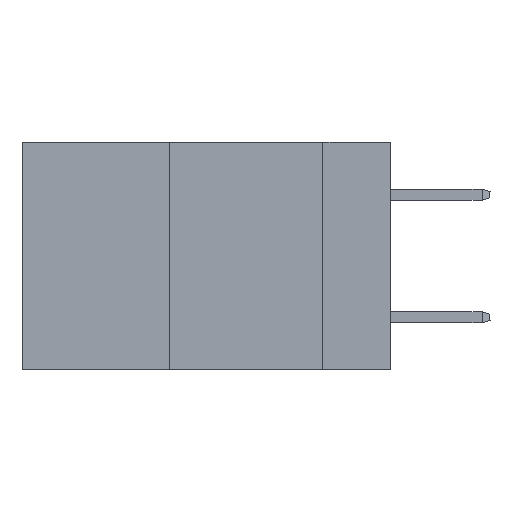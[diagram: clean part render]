
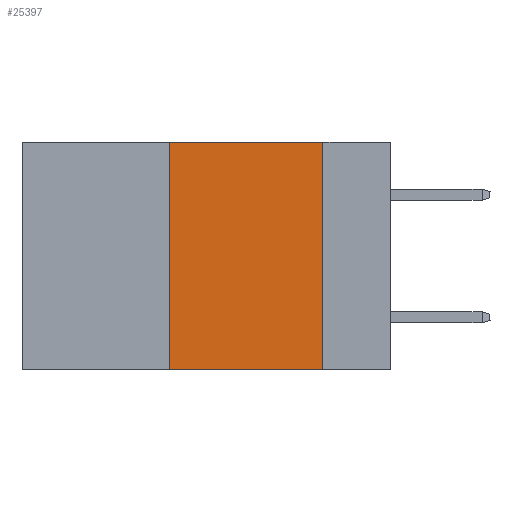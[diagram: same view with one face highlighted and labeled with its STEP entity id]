
A CAD part, left-side view. The second image highlights one B-rep face of the part: STEP entity #25397.
In plain terms, the highlighted planar face has unit normal (-1, 0, 0).
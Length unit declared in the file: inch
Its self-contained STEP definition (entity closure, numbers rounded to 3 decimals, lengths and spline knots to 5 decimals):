
#1803 = EDGE_CURVE ( 'NONE', #4967, #12010, #22935, .T. ) ;
#2272 = EDGE_CURVE ( 'NONE', #4967, #14775, #14250, .T. ) ;
#2519 = CARTESIAN_POINT ( 'NONE',  ( 0., 0.36, 0. ) ) ;
#2523 = PLANE ( 'NONE',  #8735 ) ;
#2873 = DIRECTION ( 'NONE',  ( 0., 0., -1. ) ) ;
#3216 = VECTOR ( 'NONE', #13136, 39.37008 ) ;
#4303 = ORIENTED_EDGE ( 'NONE', *, *, #10411, .F. ) ;
#4967 = VERTEX_POINT ( 'NONE', #12943 ) ;
#6997 = CARTESIAN_POINT ( 'NONE',  ( 0., 0.11, -0.37 ) ) ;
#7679 = EDGE_CURVE ( 'NONE', #14775, #32514, #18410, .T. ) ;
#8004 = ORIENTED_EDGE ( 'NONE', *, *, #7679, .F. ) ;
#8735 = AXIS2_PLACEMENT_3D ( 'NONE', #20951, #15665, #33704 ) ;
#10411 = EDGE_CURVE ( 'NONE', #32514, #12010, #24286, .T. ) ;
#10512 = CARTESIAN_POINT ( 'NONE',  ( 0., 0.11, 0. ) ) ;
#12010 = VERTEX_POINT ( 'NONE', #6997 ) ;
#12943 = CARTESIAN_POINT ( 'NONE',  ( 0., 0.36, -0.37 ) ) ;
#13136 = DIRECTION ( 'NONE',  ( 0., 0., 1. ) ) ;
#13449 = VECTOR ( 'NONE', #31368, 39.37008 ) ;
#14250 = LINE ( 'NONE', #2519, #3216 ) ;
#14536 = ORIENTED_EDGE ( 'NONE', *, *, #1803, .T. ) ;
#14775 = VERTEX_POINT ( 'NONE', #26306 ) ;
#14828 = CARTESIAN_POINT ( 'NONE',  ( 0., 0.6, 0. ) ) ;
#14901 = FACE_OUTER_BOUND ( 'NONE', #33478, .T. ) ;
#15665 = DIRECTION ( 'NONE',  ( 1., 0., 0. ) ) ;
#18410 = LINE ( 'NONE', #14828, #22144 ) ;
#20099 = DIRECTION ( 'NONE',  ( 0., -1., 0. ) ) ;
#20951 = CARTESIAN_POINT ( 'NONE',  ( 0., 0.6, 0. ) ) ;
#22144 = VECTOR ( 'NONE', #20099, 39.37008 ) ;
#22935 = LINE ( 'NONE', #33199, #13449 ) ;
#24286 = LINE ( 'NONE', #10512, #27549 ) ;
#25397 = ADVANCED_FACE ( 'NONE', ( #14901 ), #2523, .F. ) ;
#26306 = CARTESIAN_POINT ( 'NONE',  ( 0., 0.36, 0. ) ) ;
#27549 = VECTOR ( 'NONE', #2873, 39.37008 ) ;
#30855 = ORIENTED_EDGE ( 'NONE', *, *, #2272, .F. ) ;
#31368 = DIRECTION ( 'NONE',  ( 0., -1., 0. ) ) ;
#32514 = VERTEX_POINT ( 'NONE', #33108 ) ;
#33108 = CARTESIAN_POINT ( 'NONE',  ( 0., 0.11, 0. ) ) ;
#33199 = CARTESIAN_POINT ( 'NONE',  ( 0., 0.6, -0.37 ) ) ;
#33478 = EDGE_LOOP ( 'NONE', ( #4303, #8004, #30855, #14536 ) ) ;
#33704 = DIRECTION ( 'NONE',  ( 0., 0., -1. ) ) ;
